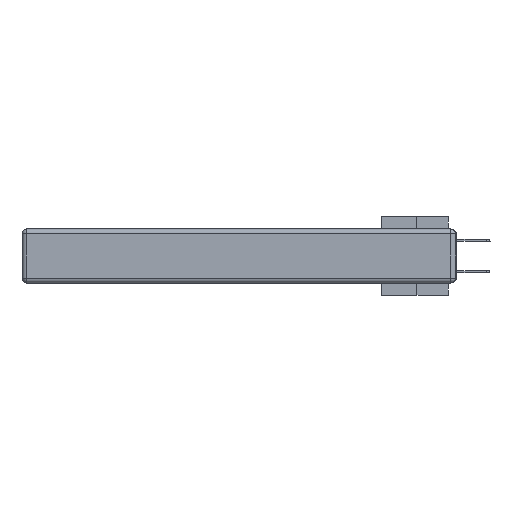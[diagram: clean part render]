
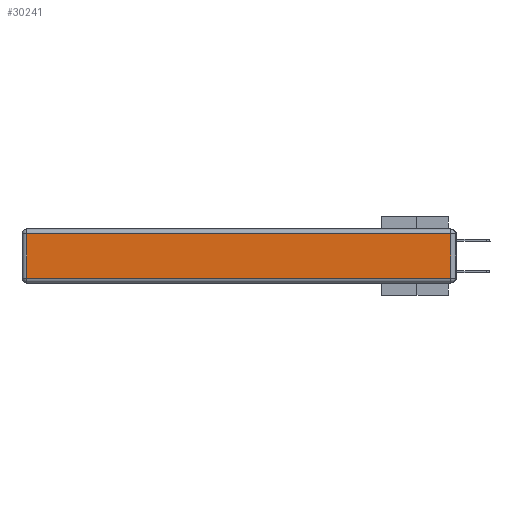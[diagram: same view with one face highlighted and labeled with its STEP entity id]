
A CAD part, left-side view. The second image highlights one B-rep face of the part: STEP entity #30241.
In plain terms, the highlighted planar face has unit normal (-1, 0, 0).
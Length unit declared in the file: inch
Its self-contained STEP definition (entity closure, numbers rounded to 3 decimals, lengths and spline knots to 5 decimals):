
#1046 = VERTEX_POINT ( 'NONE', #20941 ) ;
#1397 = PLANE ( 'NONE',  #12116 ) ;
#2144 = ORIENTED_EDGE ( 'NONE', *, *, #6172, .T. ) ;
#3723 = DIRECTION ( 'NONE',  ( 0., -1., 0. ) ) ;
#4149 = VERTEX_POINT ( 'NONE', #29053 ) ;
#5139 = LINE ( 'NONE', #19474, #35223 ) ;
#6111 = DIRECTION ( 'NONE',  ( 0., 0., 1. ) ) ;
#6172 = EDGE_CURVE ( 'NONE', #11421, #1046, #25281, .T. ) ;
#8748 = ORIENTED_EDGE ( 'NONE', *, *, #10210, .T. ) ;
#10210 = EDGE_CURVE ( 'NONE', #1046, #4149, #21622, .T. ) ;
#10366 = DIRECTION ( 'NONE',  ( 0., 0., 1. ) ) ;
#11421 = VERTEX_POINT ( 'NONE', #37716 ) ;
#12116 = AXIS2_PLACEMENT_3D ( 'NONE', #22452, #36825, #10366 ) ;
#13064 = VERTEX_POINT ( 'NONE', #16112 ) ;
#13227 = ORIENTED_EDGE ( 'NONE', *, *, #22907, .T. ) ;
#13446 = VECTOR ( 'NONE', #6111, 39.37008 ) ;
#16112 = CARTESIAN_POINT ( 'NONE',  ( 0., 2.72, -0.313 ) ) ;
#19474 = CARTESIAN_POINT ( 'NONE',  ( 0., 2.72, -0.343 ) ) ;
#20127 = DIRECTION ( 'NONE',  ( 0., 1., 0. ) ) ;
#20941 = CARTESIAN_POINT ( 'NONE',  ( 0., 0.03, -0.03 ) ) ;
#21622 = LINE ( 'NONE', #34374, #24324 ) ;
#22399 = EDGE_CURVE ( 'NONE', #13064, #11421, #25241, .T. ) ;
#22452 = CARTESIAN_POINT ( 'NONE',  ( 0., 0., -0.343 ) ) ;
#22907 = EDGE_CURVE ( 'NONE', #4149, #13064, #5139, .T. ) ;
#23572 = CARTESIAN_POINT ( 'NONE',  ( 0., 0.03, -0.343 ) ) ;
#24324 = VECTOR ( 'NONE', #20127, 39.37008 ) ;
#24402 = CARTESIAN_POINT ( 'NONE',  ( 0., 0., -0.313 ) ) ;
#24831 = EDGE_LOOP ( 'NONE', ( #34639, #2144, #8748, #13227 ) ) ;
#25241 = LINE ( 'NONE', #24402, #34368 ) ;
#25281 = LINE ( 'NONE', #23572, #13446 ) ;
#28001 = DIRECTION ( 'NONE',  ( 0., 0., -1. ) ) ;
#29053 = CARTESIAN_POINT ( 'NONE',  ( 0., 2.72, -0.03 ) ) ;
#30241 = ADVANCED_FACE ( 'NONE', ( #37425 ), #1397, .T. ) ;
#34368 = VECTOR ( 'NONE', #3723, 39.37008 ) ;
#34374 = CARTESIAN_POINT ( 'NONE',  ( 0., 2.75, -0.03 ) ) ;
#34639 = ORIENTED_EDGE ( 'NONE', *, *, #22399, .T. ) ;
#35223 = VECTOR ( 'NONE', #28001, 39.37008 ) ;
#36825 = DIRECTION ( 'NONE',  ( -1., 0., 0. ) ) ;
#37425 = FACE_OUTER_BOUND ( 'NONE', #24831, .T. ) ;
#37716 = CARTESIAN_POINT ( 'NONE',  ( 0., 0.03, -0.313 ) ) ;
